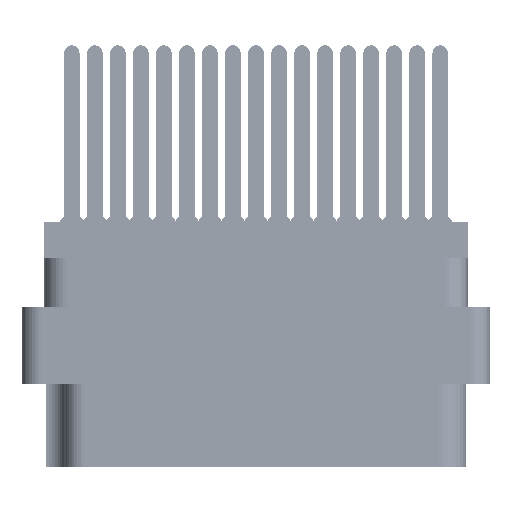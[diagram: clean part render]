
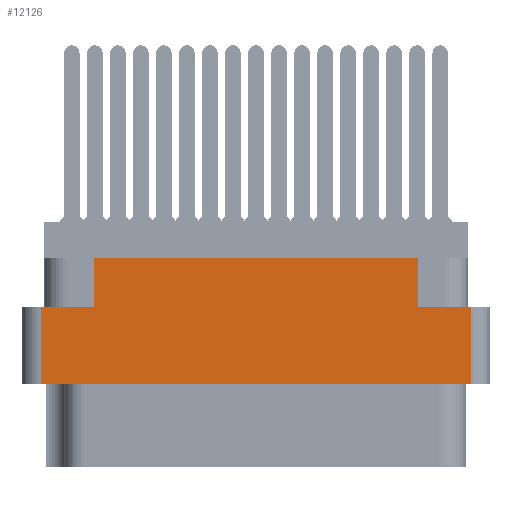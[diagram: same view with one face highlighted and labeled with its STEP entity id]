
A CAD part, left-side view. The second image highlights one B-rep face of the part: STEP entity #12126.
In plain terms, the highlighted planar face has unit normal (-1, 0, 0).
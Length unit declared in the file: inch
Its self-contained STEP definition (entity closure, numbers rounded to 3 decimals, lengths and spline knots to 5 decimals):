
#848 = CARTESIAN_POINT ( 'NONE',  ( -1.375, 0., -0.277 ) ) ;
#2886 = DIRECTION ( 'NONE',  ( 0., 0., 1. ) ) ;
#2989 = ORIENTED_EDGE ( 'NONE', *, *, #6126, .F. ) ;
#3314 = ORIENTED_EDGE ( 'NONE', *, *, #10309, .F. ) ;
#4577 = DIRECTION ( 'NONE',  ( 0., 0., 1. ) ) ;
#4887 = CARTESIAN_POINT ( 'NONE',  ( -1.375, -0.5285, -0.277 ) ) ;
#6126 = EDGE_CURVE ( 'NONE', #89336, #18086, #35977, .T. ) ;
#7745 = CARTESIAN_POINT ( 'NONE',  ( -1.375, 0., -0.529 ) ) ;
#8305 = LINE ( 'NONE', #848, #45578 ) ;
#10309 = EDGE_CURVE ( 'NONE', #42447, #65577, #12035, .T. ) ;
#12035 = LINE ( 'NONE', #7745, #44923 ) ;
#12126 = ADVANCED_FACE ( 'NONE', ( #50093 ), #78361, .T. ) ;
#12302 = VECTOR ( 'NONE', #67840, 39.37008 ) ;
#18086 = VERTEX_POINT ( 'NONE', #82048 ) ;
#18105 = CARTESIAN_POINT ( 'NONE',  ( -1.375, 0.7625, -0.117 ) ) ;
#18626 = CARTESIAN_POINT ( 'NONE',  ( -1.375, -0.7005, -0.798 ) ) ;
#19864 = EDGE_CURVE ( 'NONE', #89336, #85922, #40896, .T. ) ;
#27551 = VECTOR ( 'NONE', #42389, 39.37008 ) ;
#28452 = CARTESIAN_POINT ( 'NONE',  ( -1.375, -0.5285, -0.117 ) ) ;
#30306 = EDGE_CURVE ( 'NONE', #40853, #52799, #66904, .T. ) ;
#30585 = VERTEX_POINT ( 'NONE', #66707 ) ;
#31003 = LINE ( 'NONE', #18626, #46327 ) ;
#31482 = AXIS2_PLACEMENT_3D ( 'NONE', #73766, #72846, #2886 ) ;
#31955 = DIRECTION ( 'NONE',  ( 0., -1., 0. ) ) ;
#34735 = EDGE_CURVE ( 'NONE', #30585, #65577, #89397, .T. ) ;
#35977 = LINE ( 'NONE', #81754, #84098 ) ;
#38447 = ORIENTED_EDGE ( 'NONE', *, *, #19864, .T. ) ;
#38938 = DIRECTION ( 'NONE',  ( 0., -1., 0. ) ) ;
#40853 = VERTEX_POINT ( 'NONE', #72850 ) ;
#40896 = LINE ( 'NONE', #4887, #12302 ) ;
#42389 = DIRECTION ( 'NONE',  ( 0., 0., 1. ) ) ;
#42447 = VERTEX_POINT ( 'NONE', #88307 ) ;
#42909 = VECTOR ( 'NONE', #38938, 39.37008 ) ;
#44923 = VECTOR ( 'NONE', #70979, 39.37008 ) ;
#45578 = VECTOR ( 'NONE', #50132, 39.37008 ) ;
#46327 = VECTOR ( 'NONE', #4577, 39.37008 ) ;
#48821 = EDGE_LOOP ( 'NONE', ( #70619, #89737, #3314, #87538, #2989, #38447, #65438, #81125 ) ) ;
#49830 = EDGE_CURVE ( 'NONE', #42447, #18086, #31003, .T. ) ;
#50093 = FACE_OUTER_BOUND ( 'NONE', #48821, .T. ) ;
#50132 = DIRECTION ( 'NONE',  ( 0., -1., 0. ) ) ;
#51209 = CARTESIAN_POINT ( 'NONE',  ( -1.375, 0.5285, -0.117 ) ) ;
#51602 = LINE ( 'NONE', #18105, #42909 ) ;
#52288 = VECTOR ( 'NONE', #73068, 39.37008 ) ;
#52799 = VERTEX_POINT ( 'NONE', #51209 ) ;
#53997 = EDGE_CURVE ( 'NONE', #30585, #40853, #8305, .T. ) ;
#57029 = CARTESIAN_POINT ( 'NONE',  ( -1.375, 0.5285, -0.277 ) ) ;
#61076 = CARTESIAN_POINT ( 'NONE',  ( -1.375, 0.7005, -0.529 ) ) ;
#65438 = ORIENTED_EDGE ( 'NONE', *, *, #80405, .F. ) ;
#65577 = VERTEX_POINT ( 'NONE', #61076 ) ;
#66707 = CARTESIAN_POINT ( 'NONE',  ( -1.375, 0.7005, -0.277 ) ) ;
#66904 = LINE ( 'NONE', #57029, #27551 ) ;
#67840 = DIRECTION ( 'NONE',  ( 0., 0., 1. ) ) ;
#70619 = ORIENTED_EDGE ( 'NONE', *, *, #53997, .F. ) ;
#70767 = CARTESIAN_POINT ( 'NONE',  ( -1.375, -0.5285, -0.277 ) ) ;
#70979 = DIRECTION ( 'NONE',  ( 0., 1., 0. ) ) ;
#72846 = DIRECTION ( 'NONE',  ( -1., 0., 0. ) ) ;
#72850 = CARTESIAN_POINT ( 'NONE',  ( -1.375, 0.5285, -0.277 ) ) ;
#73068 = DIRECTION ( 'NONE',  ( 0., 0., -1. ) ) ;
#73766 = CARTESIAN_POINT ( 'NONE',  ( -1.375, -0.7625, -0.798 ) ) ;
#78361 = PLANE ( 'NONE',  #31482 ) ;
#79488 = CARTESIAN_POINT ( 'NONE',  ( -1.375, 0.7005, -0.798 ) ) ;
#80405 = EDGE_CURVE ( 'NONE', #52799, #85922, #51602, .T. ) ;
#81125 = ORIENTED_EDGE ( 'NONE', *, *, #30306, .F. ) ;
#81754 = CARTESIAN_POINT ( 'NONE',  ( -1.375, 0., -0.277 ) ) ;
#82048 = CARTESIAN_POINT ( 'NONE',  ( -1.375, -0.7005, -0.277 ) ) ;
#84098 = VECTOR ( 'NONE', #31955, 39.37008 ) ;
#85922 = VERTEX_POINT ( 'NONE', #28452 ) ;
#87538 = ORIENTED_EDGE ( 'NONE', *, *, #49830, .T. ) ;
#88307 = CARTESIAN_POINT ( 'NONE',  ( -1.375, -0.7005, -0.529 ) ) ;
#89336 = VERTEX_POINT ( 'NONE', #70767 ) ;
#89397 = LINE ( 'NONE', #79488, #52288 ) ;
#89737 = ORIENTED_EDGE ( 'NONE', *, *, #34735, .T. ) ;
